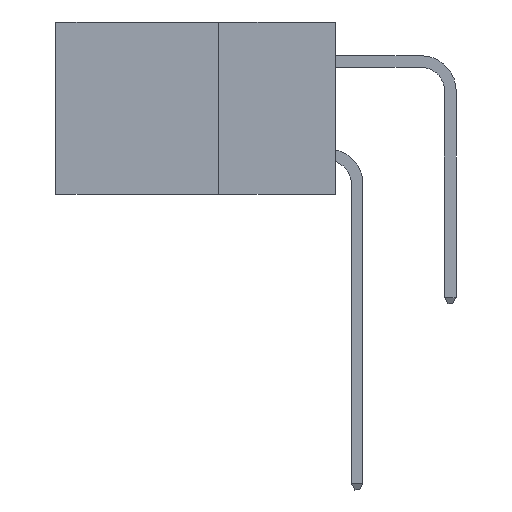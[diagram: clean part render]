
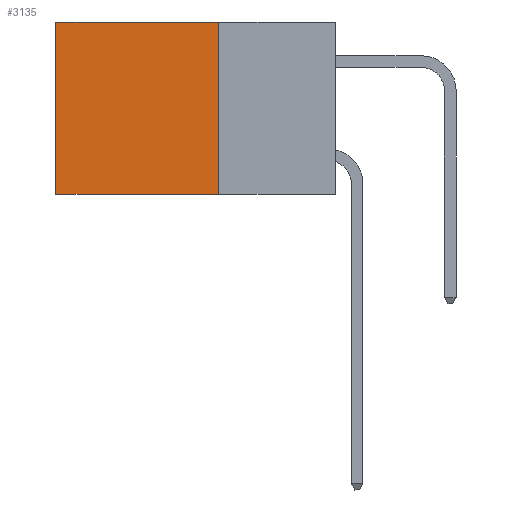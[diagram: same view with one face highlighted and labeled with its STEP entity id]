
A CAD part, left-side view. The second image highlights one B-rep face of the part: STEP entity #3135.
In plain terms, the highlighted planar face has unit normal (-1, 0, 0).
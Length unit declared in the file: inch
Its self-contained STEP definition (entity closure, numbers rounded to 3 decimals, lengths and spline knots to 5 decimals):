
#489 = DIRECTION ( 'NONE',  ( 0., 0., -1. ) ) ;
#1599 = ORIENTED_EDGE ( 'NONE', *, *, #3434, .F. ) ;
#2999 = EDGE_LOOP ( 'NONE', ( #8593, #1599, #19408, #30806 ) ) ;
#3135 = ADVANCED_FACE ( 'NONE', ( #28905 ), #12439, .F. ) ;
#3434 = EDGE_CURVE ( 'NONE', #16935, #27693, #19486, .T. ) ;
#3853 = CARTESIAN_POINT ( 'NONE',  ( 0.2875, 0.25, 0. ) ) ;
#4826 = CARTESIAN_POINT ( 'NONE',  ( 0.2875, 0.25, 0. ) ) ;
#5920 = CARTESIAN_POINT ( 'NONE',  ( 0.2875, 0.25, -0.37 ) ) ;
#6158 = VECTOR ( 'NONE', #13502, 39.37008 ) ;
#8370 = AXIS2_PLACEMENT_3D ( 'NONE', #4826, #29934, #14943 ) ;
#8582 = CARTESIAN_POINT ( 'NONE',  ( 0.2875, 0.25, -0.37 ) ) ;
#8593 = ORIENTED_EDGE ( 'NONE', *, *, #13789, .T. ) ;
#10605 = CARTESIAN_POINT ( 'NONE',  ( 0.2875, 0.6, 0. ) ) ;
#12439 = PLANE ( 'NONE',  #8370 ) ;
#12687 = LINE ( 'NONE', #3853, #18547 ) ;
#12701 = LINE ( 'NONE', #10605, #18555 ) ;
#13502 = DIRECTION ( 'NONE',  ( 0., 1., 0. ) ) ;
#13789 = EDGE_CURVE ( 'NONE', #25154, #27693, #12701, .T. ) ;
#14779 = CARTESIAN_POINT ( 'NONE',  ( 0.2875, 0.6, 0. ) ) ;
#14943 = DIRECTION ( 'NONE',  ( 0., 0., -1. ) ) ;
#16935 = VERTEX_POINT ( 'NONE', #8582 ) ;
#18547 = VECTOR ( 'NONE', #23941, 39.37008 ) ;
#18555 = VECTOR ( 'NONE', #489, 39.37008 ) ;
#18642 = DIRECTION ( 'NONE',  ( 0., 1., 0. ) ) ;
#18876 = CARTESIAN_POINT ( 'NONE',  ( 0.2875, 0.25, 0. ) ) ;
#19408 = ORIENTED_EDGE ( 'NONE', *, *, #31132, .F. ) ;
#19486 = LINE ( 'NONE', #5920, #6158 ) ;
#19548 = CARTESIAN_POINT ( 'NONE',  ( 0.2875, 0.6, -0.37 ) ) ;
#23617 = VERTEX_POINT ( 'NONE', #18876 ) ;
#23941 = DIRECTION ( 'NONE',  ( 0., 0., -1. ) ) ;
#25154 = VERTEX_POINT ( 'NONE', #14779 ) ;
#27693 = VERTEX_POINT ( 'NONE', #19548 ) ;
#28423 = VECTOR ( 'NONE', #18642, 39.37008 ) ;
#28601 = CARTESIAN_POINT ( 'NONE',  ( 0.2875, 0.25, 0. ) ) ;
#28905 = FACE_OUTER_BOUND ( 'NONE', #2999, .T. ) ;
#29226 = LINE ( 'NONE', #28601, #28423 ) ;
#29238 = EDGE_CURVE ( 'NONE', #23617, #25154, #29226, .T. ) ;
#29934 = DIRECTION ( 'NONE',  ( 1., 0., 0. ) ) ;
#30806 = ORIENTED_EDGE ( 'NONE', *, *, #29238, .T. ) ;
#31132 = EDGE_CURVE ( 'NONE', #23617, #16935, #12687, .T. ) ;
